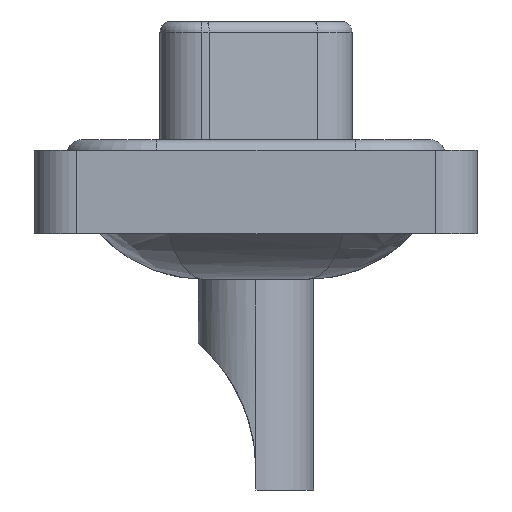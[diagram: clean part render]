
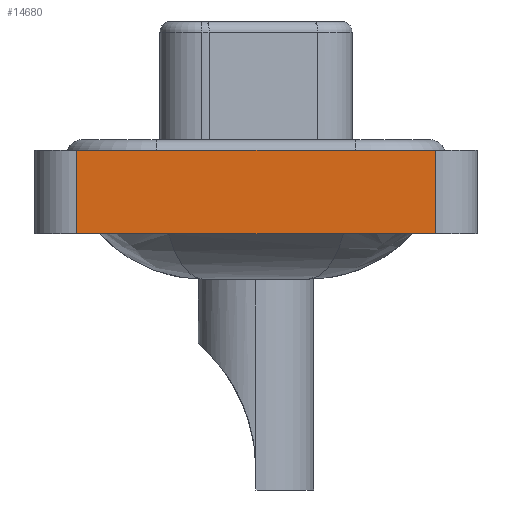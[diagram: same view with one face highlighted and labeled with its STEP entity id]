
A CAD part, left-side view. The second image highlights one B-rep face of the part: STEP entity #14680.
In plain terms, the highlighted planar face has unit normal (-1, 0, 0).
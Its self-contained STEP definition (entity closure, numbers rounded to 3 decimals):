
#131 = CARTESIAN_POINT ( 'NONE',  ( -7.35, -8.55, 0.4 ) ) ;
#378 = VERTEX_POINT ( 'NONE', #21272 ) ;
#497 = DIRECTION ( 'NONE',  ( 0., 0., 1. ) ) ;
#711 = VECTOR ( 'NONE', #5200, 1000. ) ;
#1130 = VERTEX_POINT ( 'NONE', #131 ) ;
#1583 = EDGE_CURVE ( 'NONE', #378, #6941, #15414, .T. ) ;
#1941 = LINE ( 'NONE', #15781, #10588 ) ;
#2285 = EDGE_CURVE ( 'NONE', #10203, #1130, #13837, .T. ) ;
#2511 = DIRECTION ( 'NONE',  ( -1., 0., 0. ) ) ;
#2537 = LINE ( 'NONE', #16389, #18143 ) ;
#4166 = ORIENTED_EDGE ( 'NONE', *, *, #2285, .F. ) ;
#5131 = ORIENTED_EDGE ( 'NONE', *, *, #18147, .F. ) ;
#5200 = DIRECTION ( 'NONE',  ( 0., -1., 0. ) ) ;
#6015 = ORIENTED_EDGE ( 'NONE', *, *, #1583, .T. ) ;
#6878 = VECTOR ( 'NONE', #8500, 1000. ) ;
#6941 = VERTEX_POINT ( 'NONE', #8744 ) ;
#7408 = ORIENTED_EDGE ( 'NONE', *, *, #15471, .T. ) ;
#7739 = DIRECTION ( 'NONE',  ( 0., 0., 1. ) ) ;
#8500 = DIRECTION ( 'NONE',  ( 0., -1., 0. ) ) ;
#8744 = CARTESIAN_POINT ( 'NONE',  ( -7.35, -8.55, -3.6 ) ) ;
#10203 = VERTEX_POINT ( 'NONE', #22356 ) ;
#10588 = VECTOR ( 'NONE', #16945, 1000. ) ;
#13272 = PLANE ( 'NONE',  #16367 ) ;
#13837 = LINE ( 'NONE', #18691, #711 ) ;
#14680 = ADVANCED_FACE ( 'NONE', ( #21903 ), #13272, .T. ) ;
#15414 = LINE ( 'NONE', #22224, #6878 ) ;
#15471 = EDGE_CURVE ( 'NONE', #6941, #1130, #2537, .T. ) ;
#15781 = CARTESIAN_POINT ( 'NONE',  ( -7.35, 8.55, -3.6 ) ) ;
#16367 = AXIS2_PLACEMENT_3D ( 'NONE', #20208, #2511, #7739 ) ;
#16389 = CARTESIAN_POINT ( 'NONE',  ( -7.35, -8.55, -3.6 ) ) ;
#16945 = DIRECTION ( 'NONE',  ( 0., 0., 1. ) ) ;
#18039 = EDGE_LOOP ( 'NONE', ( #7408, #4166, #5131, #6015 ) ) ;
#18143 = VECTOR ( 'NONE', #497, 1000. ) ;
#18147 = EDGE_CURVE ( 'NONE', #378, #10203, #1941, .T. ) ;
#18691 = CARTESIAN_POINT ( 'NONE',  ( -7.35, -8.55, 0.4 ) ) ;
#20208 = CARTESIAN_POINT ( 'NONE',  ( -7.35, -8.55, -3.6 ) ) ;
#21272 = CARTESIAN_POINT ( 'NONE',  ( -7.35, 8.55, -3.6 ) ) ;
#21903 = FACE_OUTER_BOUND ( 'NONE', #18039, .T. ) ;
#22224 = CARTESIAN_POINT ( 'NONE',  ( -7.35, -8.55, -3.6 ) ) ;
#22356 = CARTESIAN_POINT ( 'NONE',  ( -7.35, 8.55, 0.4 ) ) ;
